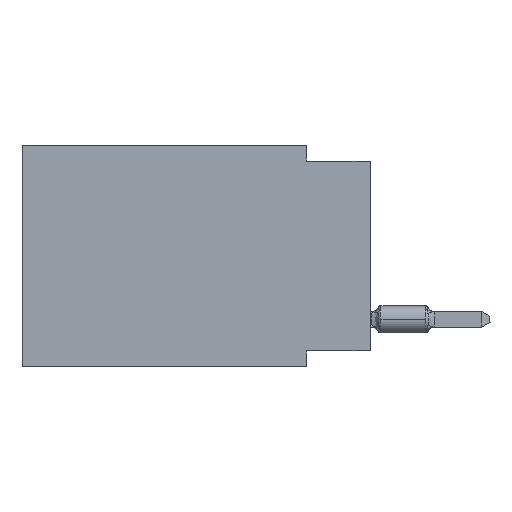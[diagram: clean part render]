
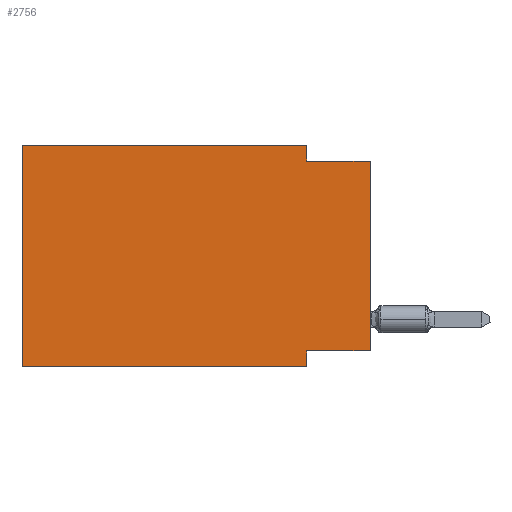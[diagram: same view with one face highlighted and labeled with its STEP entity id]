
A CAD part, left-side view. The second image highlights one B-rep face of the part: STEP entity #2756.
In plain terms, the highlighted planar face has unit normal (-1, 0, 0).
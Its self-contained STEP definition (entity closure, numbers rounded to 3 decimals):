
#124 = CARTESIAN_POINT ( 'NONE',  ( 0., 13.97, 0. ) ) ;
#376 = LINE ( 'NONE', #9460, #19951 ) ;
#560 = EDGE_CURVE ( 'NONE', #6389, #24171, #15591, .T. ) ;
#1152 = DIRECTION ( 'NONE',  ( 0., 0., -1. ) ) ;
#1538 = DIRECTION ( 'NONE',  ( 0., 0., -1. ) ) ;
#1621 = ORIENTED_EDGE ( 'NONE', *, *, #16591, .F. ) ;
#2021 = CARTESIAN_POINT ( 'NONE',  ( 0., 2.54, -8.255 ) ) ;
#2090 = DIRECTION ( 'NONE',  ( 0., 1., 0. ) ) ;
#2364 = LINE ( 'NONE', #17454, #14845 ) ;
#2756 = ADVANCED_FACE ( 'NONE', ( #4589 ), #13934, .F. ) ;
#2984 = VERTEX_POINT ( 'NONE', #11202 ) ;
#3116 = CARTESIAN_POINT ( 'NONE',  ( 0., 2.54, 0. ) ) ;
#3259 = LINE ( 'NONE', #20087, #10382 ) ;
#3703 = EDGE_LOOP ( 'NONE', ( #23673, #1621, #14715, #6832, #24264, #13432, #18481, #13786 ) ) ;
#4163 = DIRECTION ( 'NONE',  ( 0., 0., 1. ) ) ;
#4335 = CARTESIAN_POINT ( 'NONE',  ( 0., 0., -8.255 ) ) ;
#4345 = CARTESIAN_POINT ( 'NONE',  ( 0., 13.97, 0. ) ) ;
#4589 = FACE_OUTER_BOUND ( 'NONE', #3703, .T. ) ;
#4922 = DIRECTION ( 'NONE',  ( 0., 0., 1. ) ) ;
#5176 = DIRECTION ( 'NONE',  ( 0., -1., 0. ) ) ;
#5443 = CARTESIAN_POINT ( 'NONE',  ( 0., 2.54, 0. ) ) ;
#6389 = VERTEX_POINT ( 'NONE', #8583 ) ;
#6581 = VECTOR ( 'NONE', #1152, 1000. ) ;
#6832 = ORIENTED_EDGE ( 'NONE', *, *, #18690, .F. ) ;
#7119 = LINE ( 'NONE', #14617, #23145 ) ;
#7131 = CARTESIAN_POINT ( 'NONE',  ( 0., 0., -0.635 ) ) ;
#7630 = DIRECTION ( 'NONE',  ( 0., -1., 0. ) ) ;
#8157 = VECTOR ( 'NONE', #10288, 1000. ) ;
#8549 = LINE ( 'NONE', #23287, #8157 ) ;
#8583 = CARTESIAN_POINT ( 'NONE',  ( 0., 13.97, -8.89 ) ) ;
#8633 = LINE ( 'NONE', #3116, #6581 ) ;
#9057 = VERTEX_POINT ( 'NONE', #12931 ) ;
#9460 = CARTESIAN_POINT ( 'NONE',  ( 0., 0., -8.255 ) ) ;
#9760 = VECTOR ( 'NONE', #5176, 1000. ) ;
#9922 = VERTEX_POINT ( 'NONE', #2021 ) ;
#10073 = LINE ( 'NONE', #7131, #9760 ) ;
#10288 = DIRECTION ( 'NONE',  ( 0., -1., 0. ) ) ;
#10382 = VECTOR ( 'NONE', #1538, 1000. ) ;
#11202 = CARTESIAN_POINT ( 'NONE',  ( 0., 0., -0.635 ) ) ;
#12026 = VERTEX_POINT ( 'NONE', #18840 ) ;
#12033 = VERTEX_POINT ( 'NONE', #4335 ) ;
#12931 = CARTESIAN_POINT ( 'NONE',  ( 0., 2.54, -8.89 ) ) ;
#13432 = ORIENTED_EDGE ( 'NONE', *, *, #16051, .T. ) ;
#13786 = ORIENTED_EDGE ( 'NONE', *, *, #16551, .F. ) ;
#13934 = PLANE ( 'NONE',  #23554 ) ;
#14028 = VECTOR ( 'NONE', #4163, 1000. ) ;
#14617 = CARTESIAN_POINT ( 'NONE',  ( 0., 0., 0. ) ) ;
#14680 = CARTESIAN_POINT ( 'NONE',  ( 0., 13.97, 0. ) ) ;
#14715 = ORIENTED_EDGE ( 'NONE', *, *, #19053, .F. ) ;
#14845 = VECTOR ( 'NONE', #7630, 1000. ) ;
#15591 = LINE ( 'NONE', #124, #14028 ) ;
#16051 = EDGE_CURVE ( 'NONE', #6389, #9057, #2364, .T. ) ;
#16551 = EDGE_CURVE ( 'NONE', #12033, #9922, #376, .T. ) ;
#16591 = EDGE_CURVE ( 'NONE', #12026, #2984, #10073, .T. ) ;
#17454 = CARTESIAN_POINT ( 'NONE',  ( 0., 13.97, -8.89 ) ) ;
#18481 = ORIENTED_EDGE ( 'NONE', *, *, #23029, .F. ) ;
#18690 = EDGE_CURVE ( 'NONE', #24171, #19244, #8549, .T. ) ;
#18840 = CARTESIAN_POINT ( 'NONE',  ( 0., 2.54, -0.635 ) ) ;
#19053 = EDGE_CURVE ( 'NONE', #19244, #12026, #8633, .T. ) ;
#19244 = VERTEX_POINT ( 'NONE', #5443 ) ;
#19573 = DIRECTION ( 'NONE',  ( 1., 0., 0. ) ) ;
#19951 = VECTOR ( 'NONE', #2090, 1000. ) ;
#20087 = CARTESIAN_POINT ( 'NONE',  ( 0., 2.54, -8.89 ) ) ;
#21634 = DIRECTION ( 'NONE',  ( 0., 0., -1. ) ) ;
#21883 = EDGE_CURVE ( 'NONE', #12033, #2984, #7119, .T. ) ;
#23029 = EDGE_CURVE ( 'NONE', #9922, #9057, #3259, .T. ) ;
#23145 = VECTOR ( 'NONE', #4922, 1000. ) ;
#23287 = CARTESIAN_POINT ( 'NONE',  ( 0., 13.97, 0. ) ) ;
#23554 = AXIS2_PLACEMENT_3D ( 'NONE', #4345, #19573, #21634 ) ;
#23673 = ORIENTED_EDGE ( 'NONE', *, *, #21883, .T. ) ;
#24171 = VERTEX_POINT ( 'NONE', #14680 ) ;
#24264 = ORIENTED_EDGE ( 'NONE', *, *, #560, .F. ) ;
